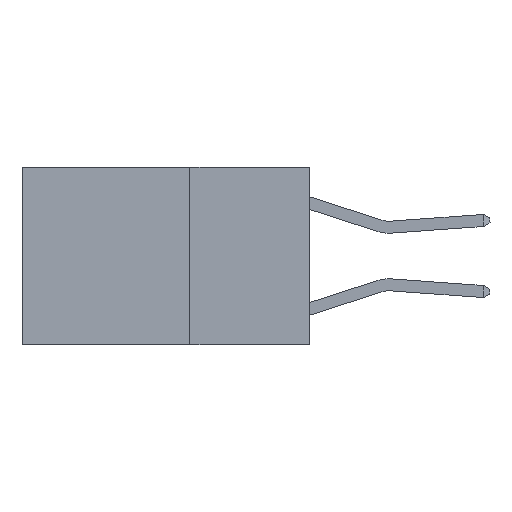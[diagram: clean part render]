
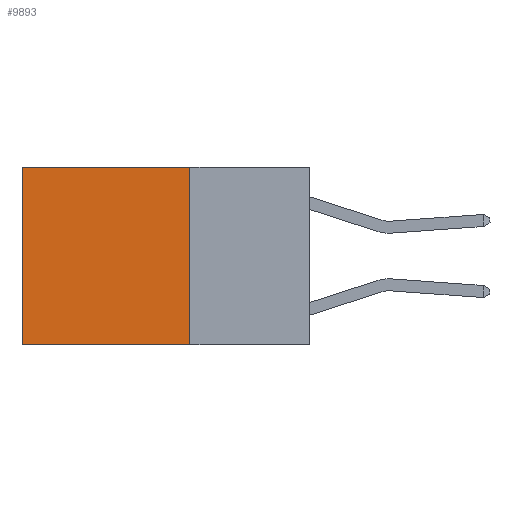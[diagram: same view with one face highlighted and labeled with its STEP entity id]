
A CAD part, left-side view. The second image highlights one B-rep face of the part: STEP entity #9893.
In plain terms, the highlighted planar face has unit normal (-1, 0, 0).
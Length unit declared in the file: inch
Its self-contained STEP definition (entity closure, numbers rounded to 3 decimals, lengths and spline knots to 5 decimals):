
#332 = DIRECTION ( 'NONE',  ( 0., 1., 0. ) ) ;
#1158 = EDGE_CURVE ( 'NONE', #7889, #10629, #7467, .T. ) ;
#1575 = CARTESIAN_POINT ( 'NONE',  ( 0.2625, 0.25, 0. ) ) ;
#1703 = VECTOR ( 'NONE', #1943, 39.37008 ) ;
#1848 = CARTESIAN_POINT ( 'NONE',  ( 0.2625, 0.25, 0. ) ) ;
#1943 = DIRECTION ( 'NONE',  ( 0., 0., -1. ) ) ;
#1969 = DIRECTION ( 'NONE',  ( 1., 0., 0. ) ) ;
#2150 = LINE ( 'NONE', #9860, #5713 ) ;
#2152 = CARTESIAN_POINT ( 'NONE',  ( 0.2625, 0.6, -0.37 ) ) ;
#2889 = FACE_OUTER_BOUND ( 'NONE', #13583, .T. ) ;
#3621 = CARTESIAN_POINT ( 'NONE',  ( 0.2625, 0.25, -0.37 ) ) ;
#3743 = CARTESIAN_POINT ( 'NONE',  ( 0.2625, 0.6, 0. ) ) ;
#5081 = CARTESIAN_POINT ( 'NONE',  ( 0.2625, 0.25, 0. ) ) ;
#5124 = DIRECTION ( 'NONE',  ( 0., 0., -1. ) ) ;
#5304 = EDGE_CURVE ( 'NONE', #7889, #13654, #2150, .T. ) ;
#5503 = LINE ( 'NONE', #3621, #6865 ) ;
#5713 = VECTOR ( 'NONE', #6410, 39.37008 ) ;
#6410 = DIRECTION ( 'NONE',  ( 0., 1., 0. ) ) ;
#6865 = VECTOR ( 'NONE', #332, 39.37008 ) ;
#6949 = ORIENTED_EDGE ( 'NONE', *, *, #1158, .F. ) ;
#7054 = AXIS2_PLACEMENT_3D ( 'NONE', #5081, #1969, #5124 ) ;
#7401 = CARTESIAN_POINT ( 'NONE',  ( 0.2625, 0.6, 0. ) ) ;
#7467 = LINE ( 'NONE', #1848, #1703 ) ;
#7889 = VERTEX_POINT ( 'NONE', #1575 ) ;
#9277 = ORIENTED_EDGE ( 'NONE', *, *, #10282, .F. ) ;
#9448 = PLANE ( 'NONE',  #7054 ) ;
#9621 = DIRECTION ( 'NONE',  ( 0., 0., -1. ) ) ;
#9781 = CARTESIAN_POINT ( 'NONE',  ( 0.2625, 0.25, -0.37 ) ) ;
#9860 = CARTESIAN_POINT ( 'NONE',  ( 0.2625, 0.25, 0. ) ) ;
#9893 = ADVANCED_FACE ( 'NONE', ( #2889 ), #9448, .F. ) ;
#10282 = EDGE_CURVE ( 'NONE', #10629, #13374, #5503, .T. ) ;
#10379 = VECTOR ( 'NONE', #9621, 39.37008 ) ;
#10629 = VERTEX_POINT ( 'NONE', #9781 ) ;
#11086 = ORIENTED_EDGE ( 'NONE', *, *, #5304, .T. ) ;
#13091 = ORIENTED_EDGE ( 'NONE', *, *, #13778, .T. ) ;
#13374 = VERTEX_POINT ( 'NONE', #2152 ) ;
#13583 = EDGE_LOOP ( 'NONE', ( #13091, #9277, #6949, #11086 ) ) ;
#13654 = VERTEX_POINT ( 'NONE', #3743 ) ;
#13755 = LINE ( 'NONE', #7401, #10379 ) ;
#13778 = EDGE_CURVE ( 'NONE', #13654, #13374, #13755, .T. ) ;
